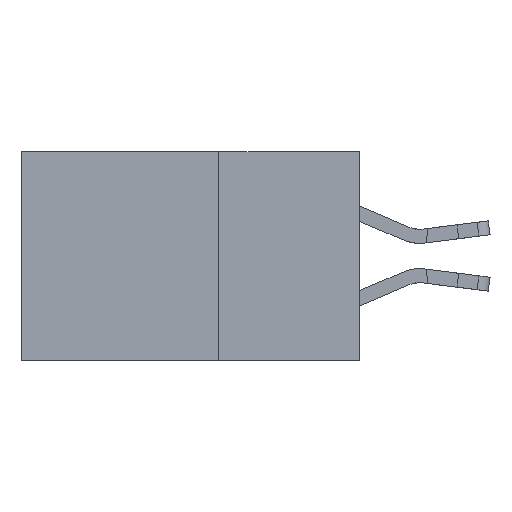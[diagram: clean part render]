
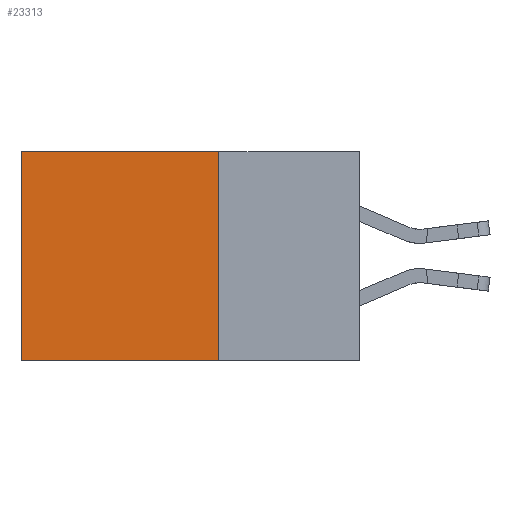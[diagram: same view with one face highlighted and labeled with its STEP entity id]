
A CAD part, left-side view. The second image highlights one B-rep face of the part: STEP entity #23313.
In plain terms, the highlighted planar face has unit normal (-1, 0, 0).
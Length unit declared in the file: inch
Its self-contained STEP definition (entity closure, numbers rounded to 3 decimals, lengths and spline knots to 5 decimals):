
#510 = VERTEX_POINT ( 'NONE', #4319 ) ;
#764 = VECTOR ( 'NONE', #14131, 39.37008 ) ;
#2773 = VERTEX_POINT ( 'NONE', #6387 ) ;
#3802 = CARTESIAN_POINT ( 'NONE',  ( 0.2875, 0.25, -0.37 ) ) ;
#4234 = LINE ( 'NONE', #26863, #19012 ) ;
#4319 = CARTESIAN_POINT ( 'NONE',  ( 0.2875, 0.25, -0.37 ) ) ;
#6387 = CARTESIAN_POINT ( 'NONE',  ( 0.2875, 0.6, -0.37 ) ) ;
#8473 = EDGE_CURVE ( 'NONE', #510, #2773, #12643, .T. ) ;
#9485 = CARTESIAN_POINT ( 'NONE',  ( 0.2875, 0.25, 0. ) ) ;
#9492 = VECTOR ( 'NONE', #12517, 39.37008 ) ;
#9580 = CARTESIAN_POINT ( 'NONE',  ( 0.2875, 0.25, 0. ) ) ;
#10604 = LINE ( 'NONE', #14745, #9492 ) ;
#12517 = DIRECTION ( 'NONE',  ( 0., 0., -1. ) ) ;
#12643 = LINE ( 'NONE', #3802, #20906 ) ;
#13580 = FACE_OUTER_BOUND ( 'NONE', #18210, .T. ) ;
#14044 = PLANE ( 'NONE',  #18374 ) ;
#14131 = DIRECTION ( 'NONE',  ( 0., 1., 0. ) ) ;
#14745 = CARTESIAN_POINT ( 'NONE',  ( 0.2875, 0.6, 0. ) ) ;
#15462 = CARTESIAN_POINT ( 'NONE',  ( 0.2875, 0.6, 0. ) ) ;
#16445 = DIRECTION ( 'NONE',  ( 0., 0., -1. ) ) ;
#16996 = EDGE_CURVE ( 'NONE', #25948, #510, #4234, .T. ) ;
#17464 = DIRECTION ( 'NONE',  ( 0., 0., -1. ) ) ;
#18210 = EDGE_LOOP ( 'NONE', ( #25496, #19406, #25164, #21600 ) ) ;
#18374 = AXIS2_PLACEMENT_3D ( 'NONE', #21082, #28081, #16445 ) ;
#19012 = VECTOR ( 'NONE', #17464, 39.37008 ) ;
#19406 = ORIENTED_EDGE ( 'NONE', *, *, #8473, .F. ) ;
#20166 = EDGE_CURVE ( 'NONE', #29286, #2773, #10604, .T. ) ;
#20906 = VECTOR ( 'NONE', #24594, 39.37008 ) ;
#21082 = CARTESIAN_POINT ( 'NONE',  ( 0.2875, 0.25, 0. ) ) ;
#21600 = ORIENTED_EDGE ( 'NONE', *, *, #25913, .T. ) ;
#23313 = ADVANCED_FACE ( 'NONE', ( #13580 ), #14044, .F. ) ;
#24594 = DIRECTION ( 'NONE',  ( 0., 1., 0. ) ) ;
#25164 = ORIENTED_EDGE ( 'NONE', *, *, #16996, .F. ) ;
#25357 = LINE ( 'NONE', #9485, #764 ) ;
#25496 = ORIENTED_EDGE ( 'NONE', *, *, #20166, .T. ) ;
#25913 = EDGE_CURVE ( 'NONE', #25948, #29286, #25357, .T. ) ;
#25948 = VERTEX_POINT ( 'NONE', #9580 ) ;
#26863 = CARTESIAN_POINT ( 'NONE',  ( 0.2875, 0.25, 0. ) ) ;
#28081 = DIRECTION ( 'NONE',  ( 1., 0., 0. ) ) ;
#29286 = VERTEX_POINT ( 'NONE', #15462 ) ;
